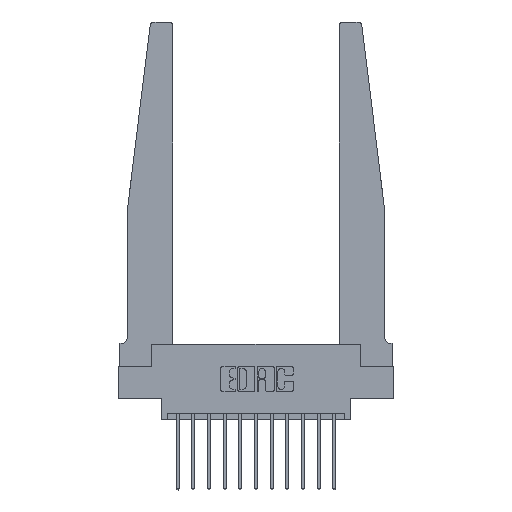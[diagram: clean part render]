
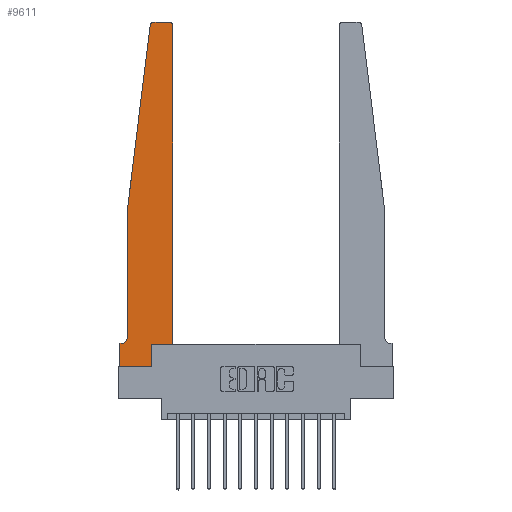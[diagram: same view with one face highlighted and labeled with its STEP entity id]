
A CAD part, top view. The second image highlights one B-rep face of the part: STEP entity #9611.
In plain terms, the highlighted planar face has unit normal (0, 0, 1).
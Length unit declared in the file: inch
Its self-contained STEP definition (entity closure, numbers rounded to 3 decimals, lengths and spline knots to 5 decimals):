
#15 = CIRCLE ( 'NONE', #2523, 0.03 ) ;
#368 = DIRECTION ( 'NONE',  ( -0.122, -0.992, 0. ) ) ;
#593 = VERTEX_POINT ( 'NONE', #5206 ) ;
#599 = EDGE_CURVE ( 'NONE', #4178, #2794, #3047, .T. ) ;
#946 = VERTEX_POINT ( 'NONE', #9585 ) ;
#1031 = CARTESIAN_POINT ( 'NONE',  ( 0.25, 2.75, 0.37 ) ) ;
#1915 = CARTESIAN_POINT ( 'NONE',  ( 0.2605, 0.18, 0.37 ) ) ;
#2050 = LINE ( 'NONE', #11666, #5443 ) ;
#2105 = CARTESIAN_POINT ( 'NONE',  ( 0.2605, 0.18, 0.37 ) ) ;
#2144 = ORIENTED_EDGE ( 'NONE', *, *, #599, .T. ) ;
#2370 = PLANE ( 'NONE',  #11863 ) ;
#2469 = LINE ( 'NONE', #1915, #12122 ) ;
#2477 = EDGE_CURVE ( 'NONE', #6984, #15361, #12966, .T. ) ;
#2523 = AXIS2_PLACEMENT_3D ( 'NONE', #13234, #5730, #14473 ) ;
#2794 = VERTEX_POINT ( 'NONE', #8716 ) ;
#2827 = ORIENTED_EDGE ( 'NONE', *, *, #5303, .T. ) ;
#2858 = CARTESIAN_POINT ( 'NONE',  ( 0.065, 0.1875, 0.37 ) ) ;
#2915 = ORIENTED_EDGE ( 'NONE', *, *, #2969, .T. ) ;
#2969 = EDGE_CURVE ( 'NONE', #593, #12955, #7047, .T. ) ;
#2987 = CARTESIAN_POINT ( 'NONE',  ( 0.27653, 2.72, 0.37 ) ) ;
#3047 = LINE ( 'NONE', #13976, #12308 ) ;
#3102 = VERTEX_POINT ( 'NONE', #10087 ) ;
#3179 = DIRECTION ( 'NONE',  ( 0., 1., 0. ) ) ;
#3265 = CARTESIAN_POINT ( 'NONE',  ( 0.425, 0.18, 0.37 ) ) ;
#3975 = CARTESIAN_POINT ( 'NONE',  ( 0.27653, 2.75, 0.37 ) ) ;
#4178 = VERTEX_POINT ( 'NONE', #2105 ) ;
#4246 = DIRECTION ( 'NONE',  ( 1., 0., 0. ) ) ;
#4495 = VECTOR ( 'NONE', #14884, 39.37008 ) ;
#4832 = ORIENTED_EDGE ( 'NONE', *, *, #15066, .T. ) ;
#4878 = ORIENTED_EDGE ( 'NONE', *, *, #2477, .T. ) ;
#4926 = DIRECTION ( 'NONE',  ( 1., 0., 0. ) ) ;
#5002 = CARTESIAN_POINT ( 'NONE',  ( 0.065, 0.2375, 0.37 ) ) ;
#5068 = ORIENTED_EDGE ( 'NONE', *, *, #16102, .T. ) ;
#5091 = VERTEX_POINT ( 'NONE', #15642 ) ;
#5206 = CARTESIAN_POINT ( 'NONE',  ( 0., 0.1875, 0.37 ) ) ;
#5217 = CARTESIAN_POINT ( 'NONE',  ( 0.065, 1.25, 0.37 ) ) ;
#5303 = EDGE_CURVE ( 'NONE', #12145, #9226, #8558, .T. ) ;
#5378 = DIRECTION ( 'NONE',  ( 0., 0., -1. ) ) ;
#5443 = VECTOR ( 'NONE', #368, 39.37008 ) ;
#5730 = DIRECTION ( 'NONE',  ( 0., 0., 1. ) ) ;
#6138 = CARTESIAN_POINT ( 'NONE',  ( 0., 0., 0.37 ) ) ;
#6681 = DIRECTION ( 'NONE',  ( 1., 0., 0. ) ) ;
#6782 = CIRCLE ( 'NONE', #10849, 0.03 ) ;
#6984 = VERTEX_POINT ( 'NONE', #5217 ) ;
#7024 = DIRECTION ( 'NONE',  ( 0., 1., 0. ) ) ;
#7047 = LINE ( 'NONE', #6138, #4495 ) ;
#7957 = AXIS2_PLACEMENT_3D ( 'NONE', #12882, #5378, #14137 ) ;
#8558 = LINE ( 'NONE', #1031, #11904 ) ;
#8651 = CARTESIAN_POINT ( 'NONE',  ( 0., 0.1875, 0.37 ) ) ;
#8716 = CARTESIAN_POINT ( 'NONE',  ( 0.425, 0.18, 0.37 ) ) ;
#9226 = VERTEX_POINT ( 'NONE', #3975 ) ;
#9249 = EDGE_CURVE ( 'NONE', #15361, #3102, #12199, .T. ) ;
#9578 = ORIENTED_EDGE ( 'NONE', *, *, #12404, .T. ) ;
#9585 = CARTESIAN_POINT ( 'NONE',  ( 0.24675, 2.72367, 0.37 ) ) ;
#9611 = ADVANCED_FACE ( 'NONE', ( #10416 ), #2370, .T. ) ;
#9619 = VECTOR ( 'NONE', #10198, 39.37008 ) ;
#9714 = ORIENTED_EDGE ( 'NONE', *, *, #12920, .T. ) ;
#9904 = VECTOR ( 'NONE', #6681, 39.37008 ) ;
#9916 = VERTEX_POINT ( 'NONE', #14540 ) ;
#10087 = CARTESIAN_POINT ( 'NONE',  ( 0.015, 0.1875, 0.37 ) ) ;
#10198 = DIRECTION ( 'NONE',  ( 0., -1., 0. ) ) ;
#10416 = FACE_OUTER_BOUND ( 'NONE', #12351, .T. ) ;
#10849 = AXIS2_PLACEMENT_3D ( 'NONE', #2987, #11808, #4246 ) ;
#11245 = ORIENTED_EDGE ( 'NONE', *, *, #14278, .T. ) ;
#11666 = CARTESIAN_POINT ( 'NONE',  ( 0.065, 1.25, 0.37 ) ) ;
#11688 = DIRECTION ( 'NONE',  ( -1., 0., 0. ) ) ;
#11808 = DIRECTION ( 'NONE',  ( 0., 0., 1. ) ) ;
#11863 = AXIS2_PLACEMENT_3D ( 'NONE', #8651, #12443, #4926 ) ;
#11904 = VECTOR ( 'NONE', #14806, 39.37008 ) ;
#12122 = VECTOR ( 'NONE', #3179, 39.37008 ) ;
#12145 = VERTEX_POINT ( 'NONE', #12772 ) ;
#12174 = ORIENTED_EDGE ( 'NONE', *, *, #9249, .T. ) ;
#12199 = CIRCLE ( 'NONE', #7957, 0.05 ) ;
#12237 = LINE ( 'NONE', #3265, #13023 ) ;
#12308 = VECTOR ( 'NONE', #15227, 39.37008 ) ;
#12351 = EDGE_LOOP ( 'NONE', ( #2827, #13725, #9714, #4878, #12174, #5068, #2915, #11245, #9578, #2144, #13426, #4832 ) ) ;
#12404 = EDGE_CURVE ( 'NONE', #5091, #4178, #2469, .T. ) ;
#12443 = DIRECTION ( 'NONE',  ( 0., 0., 1. ) ) ;
#12618 = CARTESIAN_POINT ( 'NONE',  ( 0.065, 1.25, 0.37 ) ) ;
#12772 = CARTESIAN_POINT ( 'NONE',  ( 0.395, 2.75, 0.37 ) ) ;
#12882 = CARTESIAN_POINT ( 'NONE',  ( 0.015, 0.2375, 0.37 ) ) ;
#12920 = EDGE_CURVE ( 'NONE', #946, #6984, #2050, .T. ) ;
#12929 = CARTESIAN_POINT ( 'NONE',  ( 0., 0., 0.37 ) ) ;
#12955 = VERTEX_POINT ( 'NONE', #14208 ) ;
#12966 = LINE ( 'NONE', #12618, #9619 ) ;
#13023 = VECTOR ( 'NONE', #7024, 39.37008 ) ;
#13207 = LINE ( 'NONE', #2858, #13598 ) ;
#13234 = CARTESIAN_POINT ( 'NONE',  ( 0.395, 2.72, 0.37 ) ) ;
#13238 = LINE ( 'NONE', #12929, #9904 ) ;
#13426 = ORIENTED_EDGE ( 'NONE', *, *, #15102, .T. ) ;
#13538 = EDGE_CURVE ( 'NONE', #9226, #946, #6782, .T. ) ;
#13598 = VECTOR ( 'NONE', #11688, 39.37008 ) ;
#13725 = ORIENTED_EDGE ( 'NONE', *, *, #13538, .T. ) ;
#13976 = CARTESIAN_POINT ( 'NONE',  ( 0.425, 0.18, 0.37 ) ) ;
#14137 = DIRECTION ( 'NONE',  ( -1., 0., 0. ) ) ;
#14208 = CARTESIAN_POINT ( 'NONE',  ( 0., 0., 0.37 ) ) ;
#14278 = EDGE_CURVE ( 'NONE', #12955, #5091, #13238, .T. ) ;
#14473 = DIRECTION ( 'NONE',  ( 1., 0., 0. ) ) ;
#14540 = CARTESIAN_POINT ( 'NONE',  ( 0.425, 2.72, 0.37 ) ) ;
#14806 = DIRECTION ( 'NONE',  ( -1., 0., 0. ) ) ;
#14884 = DIRECTION ( 'NONE',  ( 0., -1., 0. ) ) ;
#15066 = EDGE_CURVE ( 'NONE', #9916, #12145, #15, .T. ) ;
#15102 = EDGE_CURVE ( 'NONE', #2794, #9916, #12237, .T. ) ;
#15227 = DIRECTION ( 'NONE',  ( 1., 0., 0. ) ) ;
#15361 = VERTEX_POINT ( 'NONE', #5002 ) ;
#15642 = CARTESIAN_POINT ( 'NONE',  ( 0.2605, 0., 0.37 ) ) ;
#16102 = EDGE_CURVE ( 'NONE', #3102, #593, #13207, .T. ) ;
